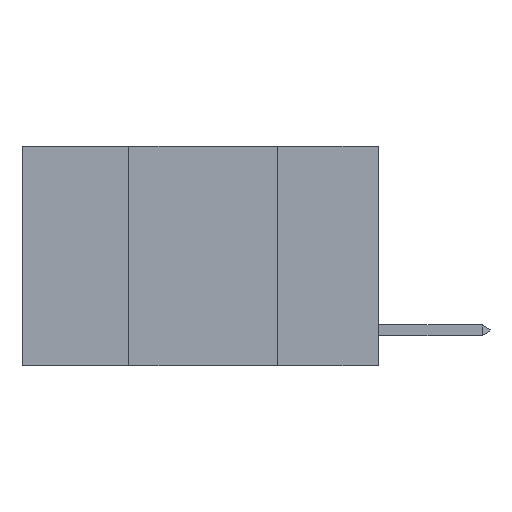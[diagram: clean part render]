
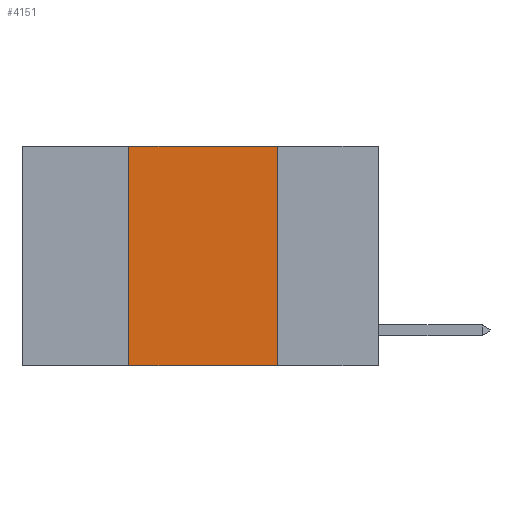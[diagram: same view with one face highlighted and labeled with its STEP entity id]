
A CAD part, left-side view. The second image highlights one B-rep face of the part: STEP entity #4151.
In plain terms, the highlighted planar face has unit normal (-1, 0, 0).
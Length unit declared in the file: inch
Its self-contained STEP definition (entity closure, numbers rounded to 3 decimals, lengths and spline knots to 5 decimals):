
#161 = DIRECTION ( 'NONE',  ( 0., 0., -1. ) ) ;
#346 = LINE ( 'NONE', #5922, #11630 ) ;
#1187 = CARTESIAN_POINT ( 'NONE',  ( 0., 0.17, 0. ) ) ;
#1614 = PLANE ( 'NONE',  #11111 ) ;
#2292 = LINE ( 'NONE', #9623, #8374 ) ;
#3055 = EDGE_CURVE ( 'NONE', #3885, #7894, #346, .T. ) ;
#3381 = LINE ( 'NONE', #8863, #7510 ) ;
#3646 = ORIENTED_EDGE ( 'NONE', *, *, #14310, .F. ) ;
#3885 = VERTEX_POINT ( 'NONE', #13015 ) ;
#3978 = VERTEX_POINT ( 'NONE', #1187 ) ;
#4151 = ADVANCED_FACE ( 'NONE', ( #12641 ), #1614, .F. ) ;
#5403 = DIRECTION ( 'NONE',  ( 0., 0., -1. ) ) ;
#5409 = DIRECTION ( 'NONE',  ( 0., -1., 0. ) ) ;
#5728 = DIRECTION ( 'NONE',  ( 1., 0., 0. ) ) ;
#5922 = CARTESIAN_POINT ( 'NONE',  ( 0., 0.6, -0.37 ) ) ;
#7510 = VECTOR ( 'NONE', #9054, 39.37008 ) ;
#7894 = VERTEX_POINT ( 'NONE', #11206 ) ;
#8374 = VECTOR ( 'NONE', #5403, 39.37008 ) ;
#8409 = VECTOR ( 'NONE', #5409, 39.37008 ) ;
#8863 = CARTESIAN_POINT ( 'NONE',  ( 0., 0.42, 0. ) ) ;
#9054 = DIRECTION ( 'NONE',  ( 0., 0., 1. ) ) ;
#9623 = CARTESIAN_POINT ( 'NONE',  ( 0., 0.17, 0. ) ) ;
#11111 = AXIS2_PLACEMENT_3D ( 'NONE', #13914, #5728, #161 ) ;
#11206 = CARTESIAN_POINT ( 'NONE',  ( 0., 0.17, -0.37 ) ) ;
#11340 = EDGE_LOOP ( 'NONE', ( #13425, #17599, #3646, #13876 ) ) ;
#11458 = DIRECTION ( 'NONE',  ( 0., -1., 0. ) ) ;
#11630 = VECTOR ( 'NONE', #11458, 39.37008 ) ;
#12037 = CARTESIAN_POINT ( 'NONE',  ( 0., 0.42, 0. ) ) ;
#12641 = FACE_OUTER_BOUND ( 'NONE', #11340, .T. ) ;
#13015 = CARTESIAN_POINT ( 'NONE',  ( 0., 0.42, -0.37 ) ) ;
#13425 = ORIENTED_EDGE ( 'NONE', *, *, #13922, .F. ) ;
#13696 = LINE ( 'NONE', #13858, #8409 ) ;
#13858 = CARTESIAN_POINT ( 'NONE',  ( 0., 0.6, 0. ) ) ;
#13876 = ORIENTED_EDGE ( 'NONE', *, *, #3055, .T. ) ;
#13914 = CARTESIAN_POINT ( 'NONE',  ( 0., 0.6, 0. ) ) ;
#13922 = EDGE_CURVE ( 'NONE', #3978, #7894, #2292, .T. ) ;
#14310 = EDGE_CURVE ( 'NONE', #3885, #15804, #3381, .T. ) ;
#15804 = VERTEX_POINT ( 'NONE', #12037 ) ;
#17146 = EDGE_CURVE ( 'NONE', #15804, #3978, #13696, .T. ) ;
#17599 = ORIENTED_EDGE ( 'NONE', *, *, #17146, .F. ) ;
